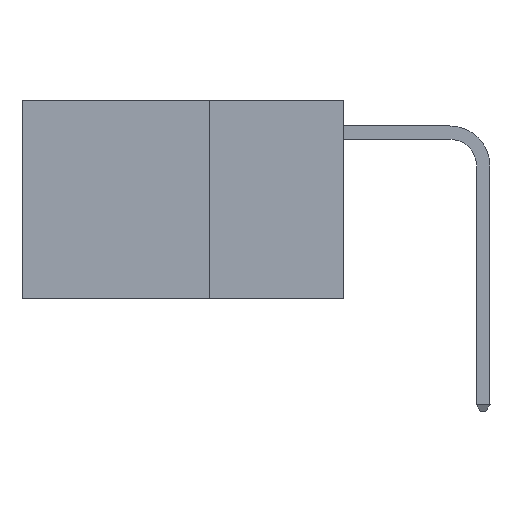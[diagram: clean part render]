
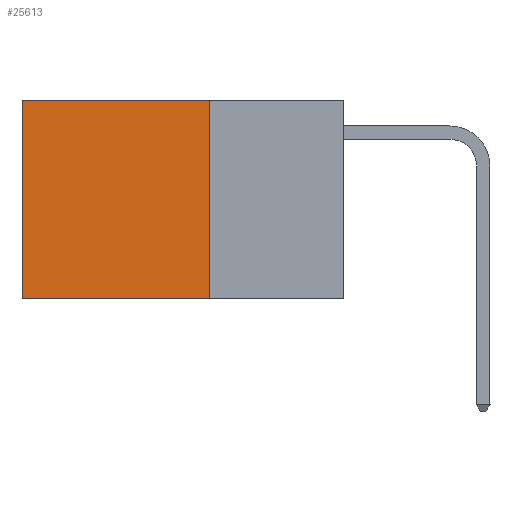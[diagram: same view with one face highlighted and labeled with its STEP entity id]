
A CAD part, left-side view. The second image highlights one B-rep face of the part: STEP entity #25613.
In plain terms, the highlighted planar face has unit normal (-1, 0, 0).
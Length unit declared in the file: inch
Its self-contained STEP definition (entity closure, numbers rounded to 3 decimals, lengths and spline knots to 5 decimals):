
#538 = CARTESIAN_POINT ( 'NONE',  ( 0.2625, 0.25, -0.37 ) ) ;
#1368 = EDGE_LOOP ( 'NONE', ( #13631, #29505, #21987, #13224 ) ) ;
#1601 = LINE ( 'NONE', #8006, #17625 ) ;
#2184 = DIRECTION ( 'NONE',  ( 1., 0., 0. ) ) ;
#3351 = VECTOR ( 'NONE', #28478, 39.37008 ) ;
#3846 = VECTOR ( 'NONE', #10502, 39.37008 ) ;
#4269 = EDGE_CURVE ( 'NONE', #29064, #22518, #12578, .T. ) ;
#5444 = VERTEX_POINT ( 'NONE', #7203 ) ;
#7203 = CARTESIAN_POINT ( 'NONE',  ( 0.2625, 0.6, -0.37 ) ) ;
#8006 = CARTESIAN_POINT ( 'NONE',  ( 0.2625, 0.25, 0. ) ) ;
#8346 = VECTOR ( 'NONE', #18322, 39.37008 ) ;
#10502 = DIRECTION ( 'NONE',  ( 0., 1., 0. ) ) ;
#12578 = LINE ( 'NONE', #19721, #3351 ) ;
#12661 = LINE ( 'NONE', #24166, #3846 ) ;
#13224 = ORIENTED_EDGE ( 'NONE', *, *, #22678, .T. ) ;
#13631 = ORIENTED_EDGE ( 'NONE', *, *, #24457, .T. ) ;
#13754 = VERTEX_POINT ( 'NONE', #20682 ) ;
#13762 = FACE_OUTER_BOUND ( 'NONE', #1368, .T. ) ;
#15449 = DIRECTION ( 'NONE',  ( 0., 1., 0. ) ) ;
#17613 = EDGE_CURVE ( 'NONE', #22518, #5444, #12661, .T. ) ;
#17625 = VECTOR ( 'NONE', #15449, 39.37008 ) ;
#18322 = DIRECTION ( 'NONE',  ( 0., 0., -1. ) ) ;
#19721 = CARTESIAN_POINT ( 'NONE',  ( 0.2625, 0.25, 0. ) ) ;
#20123 = CARTESIAN_POINT ( 'NONE',  ( 0.2625, 0.25, 0. ) ) ;
#20279 = CARTESIAN_POINT ( 'NONE',  ( 0.2625, 0.6, 0. ) ) ;
#20682 = CARTESIAN_POINT ( 'NONE',  ( 0.2625, 0.6, 0. ) ) ;
#21987 = ORIENTED_EDGE ( 'NONE', *, *, #4269, .F. ) ;
#22518 = VERTEX_POINT ( 'NONE', #538 ) ;
#22678 = EDGE_CURVE ( 'NONE', #29064, #13754, #1601, .T. ) ;
#23002 = PLANE ( 'NONE',  #27797 ) ;
#24166 = CARTESIAN_POINT ( 'NONE',  ( 0.2625, 0.25, -0.37 ) ) ;
#24457 = EDGE_CURVE ( 'NONE', #13754, #5444, #27815, .T. ) ;
#25548 = CARTESIAN_POINT ( 'NONE',  ( 0.2625, 0.25, 0. ) ) ;
#25613 = ADVANCED_FACE ( 'NONE', ( #13762 ), #23002, .F. ) ;
#27797 = AXIS2_PLACEMENT_3D ( 'NONE', #25548, #2184, #29982 ) ;
#27815 = LINE ( 'NONE', #20279, #8346 ) ;
#28478 = DIRECTION ( 'NONE',  ( 0., 0., -1. ) ) ;
#29064 = VERTEX_POINT ( 'NONE', #20123 ) ;
#29505 = ORIENTED_EDGE ( 'NONE', *, *, #17613, .F. ) ;
#29982 = DIRECTION ( 'NONE',  ( 0., 0., -1. ) ) ;
